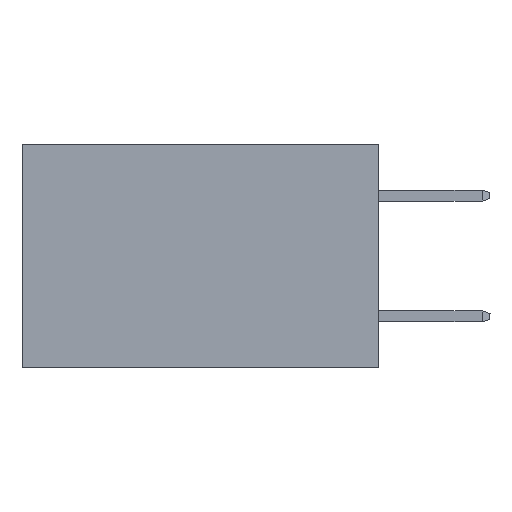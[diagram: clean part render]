
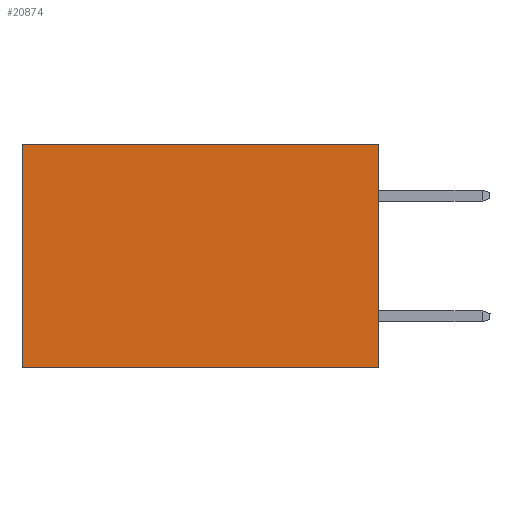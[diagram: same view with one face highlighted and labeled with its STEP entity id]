
A CAD part, left-side view. The second image highlights one B-rep face of the part: STEP entity #20874.
In plain terms, the highlighted planar face has unit normal (-1, 0, 0).
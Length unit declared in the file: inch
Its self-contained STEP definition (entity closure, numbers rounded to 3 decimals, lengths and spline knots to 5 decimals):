
#396 = CARTESIAN_POINT ( 'NONE',  ( 0.277, 0., -0.37 ) ) ;
#639 = DIRECTION ( 'NONE',  ( 0., 1., 0. ) ) ;
#709 = LINE ( 'NONE', #5811, #19010 ) ;
#802 = VECTOR ( 'NONE', #639, 39.37008 ) ;
#875 = ORIENTED_EDGE ( 'NONE', *, *, #7218, .F. ) ;
#1307 = LINE ( 'NONE', #25702, #4972 ) ;
#4327 = PLANE ( 'NONE',  #22152 ) ;
#4486 = VERTEX_POINT ( 'NONE', #8368 ) ;
#4972 = VECTOR ( 'NONE', #9587, 39.37008 ) ;
#5811 = CARTESIAN_POINT ( 'NONE',  ( 0.277, 0., 0. ) ) ;
#5874 = DIRECTION ( 'NONE',  ( 0., 0., -1. ) ) ;
#6633 = DIRECTION ( 'NONE',  ( 1., 0., 0. ) ) ;
#7218 = EDGE_CURVE ( 'NONE', #10313, #27322, #25283, .T. ) ;
#8368 = CARTESIAN_POINT ( 'NONE',  ( 0.277, 0.59, 0. ) ) ;
#9587 = DIRECTION ( 'NONE',  ( 0., 0., -1. ) ) ;
#10313 = VERTEX_POINT ( 'NONE', #25034 ) ;
#13495 = EDGE_CURVE ( 'NONE', #4486, #27322, #24679, .T. ) ;
#15061 = CARTESIAN_POINT ( 'NONE',  ( 0.277, 0., 0. ) ) ;
#15698 = VERTEX_POINT ( 'NONE', #15061 ) ;
#16096 = ORIENTED_EDGE ( 'NONE', *, *, #24599, .T. ) ;
#18725 = ORIENTED_EDGE ( 'NONE', *, *, #13495, .T. ) ;
#19010 = VECTOR ( 'NONE', #21846, 39.37008 ) ;
#19549 = CARTESIAN_POINT ( 'NONE',  ( 0.277, 0.59, -0.37 ) ) ;
#20338 = CARTESIAN_POINT ( 'NONE',  ( 0.277, 0., -0.37 ) ) ;
#20874 = ADVANCED_FACE ( 'NONE', ( #23257 ), #4327, .F. ) ;
#21753 = ORIENTED_EDGE ( 'NONE', *, *, #26346, .F. ) ;
#21846 = DIRECTION ( 'NONE',  ( 0., 1., 0. ) ) ;
#22152 = AXIS2_PLACEMENT_3D ( 'NONE', #20338, #6633, #22674 ) ;
#22674 = DIRECTION ( 'NONE',  ( 0., 0., -1. ) ) ;
#23257 = FACE_OUTER_BOUND ( 'NONE', #24185, .T. ) ;
#24185 = EDGE_LOOP ( 'NONE', ( #18725, #875, #21753, #16096 ) ) ;
#24599 = EDGE_CURVE ( 'NONE', #15698, #4486, #709, .T. ) ;
#24679 = LINE ( 'NONE', #19549, #25394 ) ;
#25034 = CARTESIAN_POINT ( 'NONE',  ( 0.277, 0., -0.37 ) ) ;
#25283 = LINE ( 'NONE', #396, #802 ) ;
#25394 = VECTOR ( 'NONE', #5874, 39.37008 ) ;
#25702 = CARTESIAN_POINT ( 'NONE',  ( 0.277, 0., -0.37 ) ) ;
#26346 = EDGE_CURVE ( 'NONE', #15698, #10313, #1307, .T. ) ;
#27322 = VERTEX_POINT ( 'NONE', #28521 ) ;
#28521 = CARTESIAN_POINT ( 'NONE',  ( 0.277, 0.59, -0.37 ) ) ;
